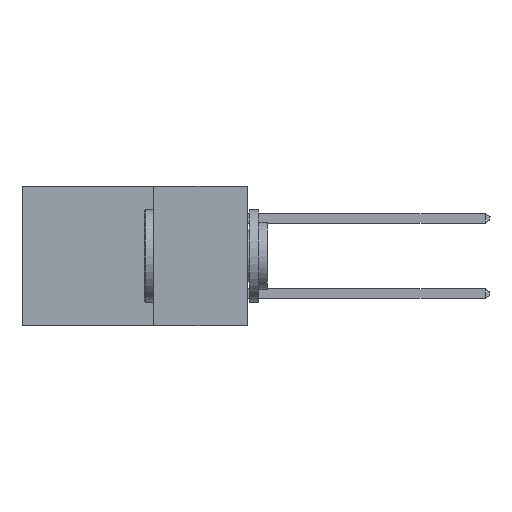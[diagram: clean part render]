
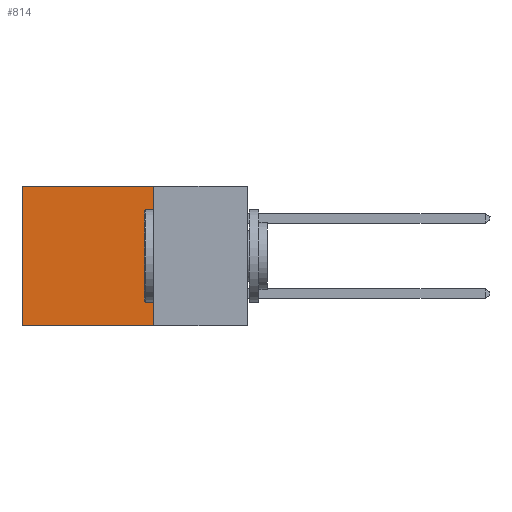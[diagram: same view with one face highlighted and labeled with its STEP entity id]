
A CAD part, left-side view. The second image highlights one B-rep face of the part: STEP entity #814.
In plain terms, the highlighted planar face has unit normal (-1, 0, 0).
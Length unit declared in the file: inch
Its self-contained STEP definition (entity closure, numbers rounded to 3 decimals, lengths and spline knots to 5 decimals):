
#519 = CARTESIAN_POINT ( 'NONE',  ( 0.2615, 0.25, 0. ) ) ;
#700 = LINE ( 'NONE', #519, #3672 ) ;
#814 = ADVANCED_FACE ( 'NONE', ( #10000 ), #5969, .F. ) ;
#873 = CARTESIAN_POINT ( 'NONE',  ( 0.2615, 0.25, -0.37 ) ) ;
#1250 = CARTESIAN_POINT ( 'NONE',  ( 0.2615, 0.25, -0.37 ) ) ;
#1479 = AXIS2_PLACEMENT_3D ( 'NONE', #12384, #9624, #13763 ) ;
#1604 = EDGE_CURVE ( 'NONE', #7015, #2243, #13837, .T. ) ;
#2243 = VERTEX_POINT ( 'NONE', #14448 ) ;
#3672 = VECTOR ( 'NONE', #9821, 39.37008 ) ;
#3706 = LINE ( 'NONE', #873, #15593 ) ;
#3903 = ORIENTED_EDGE ( 'NONE', *, *, #1604, .T. ) ;
#5515 = EDGE_LOOP ( 'NONE', ( #3903, #8007, #8198, #14399 ) ) ;
#5969 = PLANE ( 'NONE',  #1479 ) ;
#6747 = CARTESIAN_POINT ( 'NONE',  ( 0.2615, 0.25, 0. ) ) ;
#7015 = VERTEX_POINT ( 'NONE', #8254 ) ;
#7316 = LINE ( 'NONE', #1250, #16794 ) ;
#7675 = DIRECTION ( 'NONE',  ( 0., 0., -1. ) ) ;
#8007 = ORIENTED_EDGE ( 'NONE', *, *, #12146, .F. ) ;
#8013 = VERTEX_POINT ( 'NONE', #14214 ) ;
#8198 = ORIENTED_EDGE ( 'NONE', *, *, #8668, .F. ) ;
#8254 = CARTESIAN_POINT ( 'NONE',  ( 0.2615, 0.6, 0. ) ) ;
#8668 = EDGE_CURVE ( 'NONE', #9504, #8013, #3706, .T. ) ;
#9504 = VERTEX_POINT ( 'NONE', #6747 ) ;
#9624 = DIRECTION ( 'NONE',  ( 1., 0., 0. ) ) ;
#9821 = DIRECTION ( 'NONE',  ( 0., 1., 0. ) ) ;
#10000 = FACE_OUTER_BOUND ( 'NONE', #5515, .T. ) ;
#11060 = VECTOR ( 'NONE', #16370, 39.37008 ) ;
#12146 = EDGE_CURVE ( 'NONE', #8013, #2243, #7316, .T. ) ;
#12384 = CARTESIAN_POINT ( 'NONE',  ( 0.2615, 0.25, -0.37 ) ) ;
#13754 = CARTESIAN_POINT ( 'NONE',  ( 0.2615, 0.6, -0.37 ) ) ;
#13763 = DIRECTION ( 'NONE',  ( 0., 0., -1. ) ) ;
#13837 = LINE ( 'NONE', #13754, #11060 ) ;
#14214 = CARTESIAN_POINT ( 'NONE',  ( 0.2615, 0.25, -0.37 ) ) ;
#14399 = ORIENTED_EDGE ( 'NONE', *, *, #14805, .T. ) ;
#14448 = CARTESIAN_POINT ( 'NONE',  ( 0.2615, 0.6, -0.37 ) ) ;
#14805 = EDGE_CURVE ( 'NONE', #9504, #7015, #700, .T. ) ;
#15593 = VECTOR ( 'NONE', #7675, 39.37008 ) ;
#16370 = DIRECTION ( 'NONE',  ( 0., 0., -1. ) ) ;
#16794 = VECTOR ( 'NONE', #16802, 39.37008 ) ;
#16802 = DIRECTION ( 'NONE',  ( 0., 1., 0. ) ) ;
